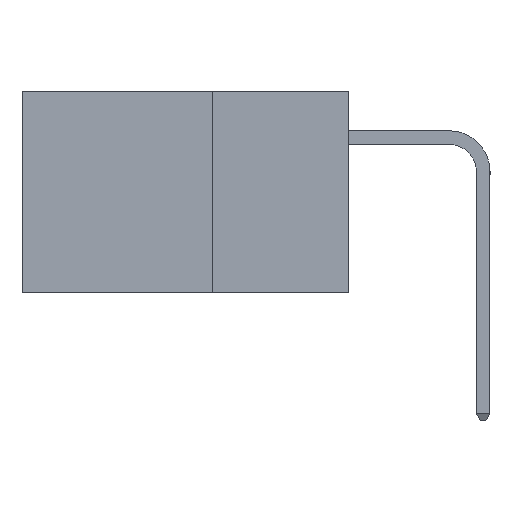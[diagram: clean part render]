
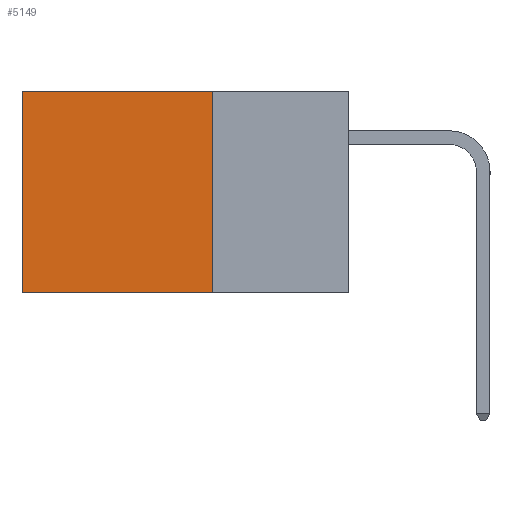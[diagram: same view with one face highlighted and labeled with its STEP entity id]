
A CAD part, left-side view. The second image highlights one B-rep face of the part: STEP entity #5149.
In plain terms, the highlighted planar face has unit normal (-1, 0, 0).
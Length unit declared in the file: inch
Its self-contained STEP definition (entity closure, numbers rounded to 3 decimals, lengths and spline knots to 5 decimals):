
#466 = VECTOR ( 'NONE', #9172, 39.37008 ) ;
#481 = EDGE_LOOP ( 'NONE', ( #5007, #9900, #8380, #5466 ) ) ;
#797 = CARTESIAN_POINT ( 'NONE',  ( 0.2875, 0.6, 0. ) ) ;
#930 = VERTEX_POINT ( 'NONE', #5931 ) ;
#976 = VERTEX_POINT ( 'NONE', #6444 ) ;
#1739 = VERTEX_POINT ( 'NONE', #4398 ) ;
#2162 = EDGE_CURVE ( 'NONE', #1739, #976, #5938, .T. ) ;
#2480 = VERTEX_POINT ( 'NONE', #6139 ) ;
#2749 = FACE_OUTER_BOUND ( 'NONE', #481, .T. ) ;
#3069 = LINE ( 'NONE', #797, #466 ) ;
#3365 = EDGE_CURVE ( 'NONE', #1739, #930, #4911, .T. ) ;
#3523 = DIRECTION ( 'NONE',  ( 1., 0., 0. ) ) ;
#3631 = DIRECTION ( 'NONE',  ( 0., 0., -1. ) ) ;
#3826 = PLANE ( 'NONE',  #5540 ) ;
#3857 = CARTESIAN_POINT ( 'NONE',  ( 0.2875, 0.25, 0. ) ) ;
#4398 = CARTESIAN_POINT ( 'NONE',  ( 0.2875, 0.25, 0. ) ) ;
#4911 = LINE ( 'NONE', #11620, #6505 ) ;
#5007 = ORIENTED_EDGE ( 'NONE', *, *, #10915, .T. ) ;
#5149 = ADVANCED_FACE ( 'NONE', ( #2749 ), #3826, .F. ) ;
#5342 = CARTESIAN_POINT ( 'NONE',  ( 0.2875, 0.25, 0. ) ) ;
#5377 = DIRECTION ( 'NONE',  ( 0., 1., 0. ) ) ;
#5466 = ORIENTED_EDGE ( 'NONE', *, *, #3365, .T. ) ;
#5540 = AXIS2_PLACEMENT_3D ( 'NONE', #3857, #3523, #3631 ) ;
#5733 = DIRECTION ( 'NONE',  ( 0., 0., -1. ) ) ;
#5931 = CARTESIAN_POINT ( 'NONE',  ( 0.2875, 0.6, 0. ) ) ;
#5938 = LINE ( 'NONE', #5342, #7768 ) ;
#6139 = CARTESIAN_POINT ( 'NONE',  ( 0.2875, 0.6, -0.37 ) ) ;
#6444 = CARTESIAN_POINT ( 'NONE',  ( 0.2875, 0.25, -0.37 ) ) ;
#6505 = VECTOR ( 'NONE', #11546, 39.37008 ) ;
#7282 = LINE ( 'NONE', #11613, #9373 ) ;
#7768 = VECTOR ( 'NONE', #5733, 39.37008 ) ;
#8380 = ORIENTED_EDGE ( 'NONE', *, *, #2162, .F. ) ;
#9172 = DIRECTION ( 'NONE',  ( 0., 0., -1. ) ) ;
#9373 = VECTOR ( 'NONE', #5377, 39.37008 ) ;
#9900 = ORIENTED_EDGE ( 'NONE', *, *, #10795, .F. ) ;
#10795 = EDGE_CURVE ( 'NONE', #976, #2480, #7282, .T. ) ;
#10915 = EDGE_CURVE ( 'NONE', #930, #2480, #3069, .T. ) ;
#11546 = DIRECTION ( 'NONE',  ( 0., 1., 0. ) ) ;
#11613 = CARTESIAN_POINT ( 'NONE',  ( 0.2875, 0.25, -0.37 ) ) ;
#11620 = CARTESIAN_POINT ( 'NONE',  ( 0.2875, 0.25, 0. ) ) ;
